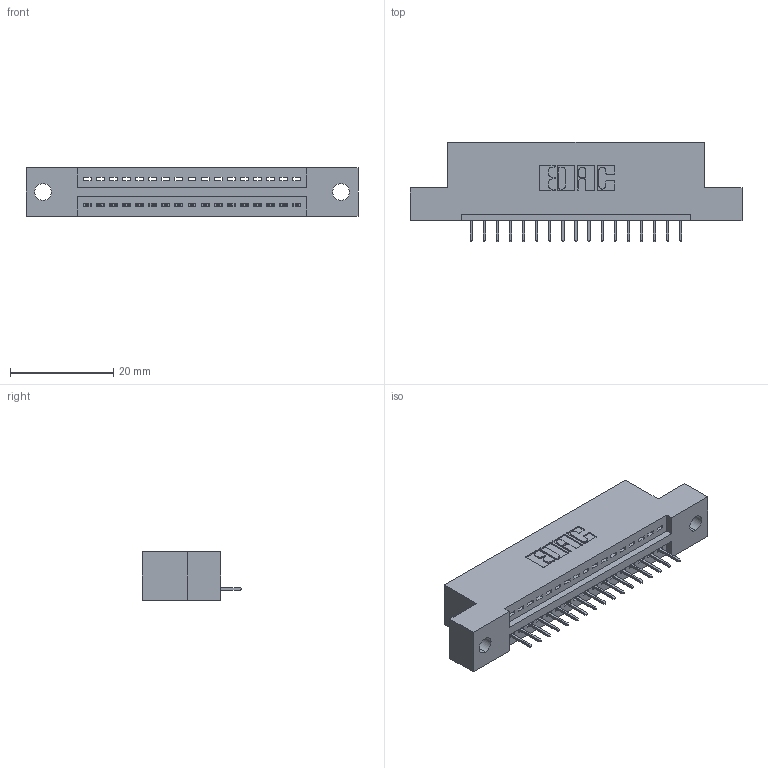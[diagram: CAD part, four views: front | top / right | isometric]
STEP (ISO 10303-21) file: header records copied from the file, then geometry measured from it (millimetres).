
FILE_DESCRIPTION (( 'STEP AP203' ), '1' );
FILE_NAME ('395-017-524-102.STEP', '2019-10-17T14:19:05', ( '' ), ( '' ), 'SwSTEP 2.0', 'SolidWorks 2016', '' );
FILE_SCHEMA (( 'CONFIG_CONTROL_DESIGN' ));
Length unit declared in the file: inch
Products named in the file (3): 395-017-524-102; 345-292-001_345-293-124; 345 Part_Flush Mounting Lugs - 0.128 Dia
Assembly tree (18 placements, depth 2):
  395-017-524-102
    345 Part_Flush Mounting Lugs - 0.128 Dia
    345-292-001_345-293-124  x17
Bounding box: 64.39 x 19.35 x 9.4 mm (x, y, z)
Volume: 5807.1 mm3; surface area: 6891.1 mm2
Topology: 18 solids, 18 shells, 1180 faces, 3401 edges, 2198 vertices
Faces by surface type: plane 862, cylinder 318
Entity records: 16237 total; most frequent: CARTESIAN_POINT 2819, ORIENTED_EDGE 2770, DIRECTION 2499, EDGE_CURVE 1385, VECTOR 1189, LINE 1189, VERTEX_POINT 918, AXIS2_PLACEMENT_3D 655
